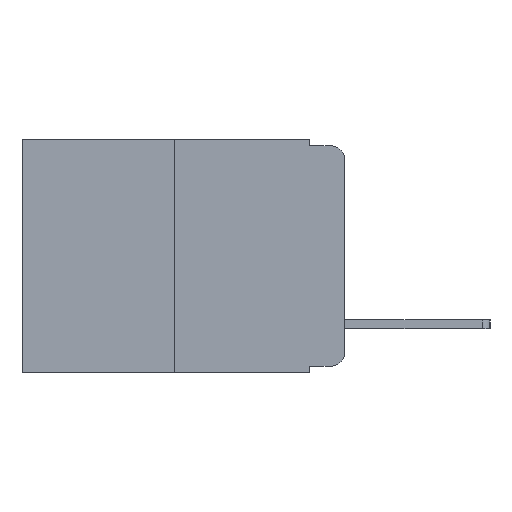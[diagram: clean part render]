
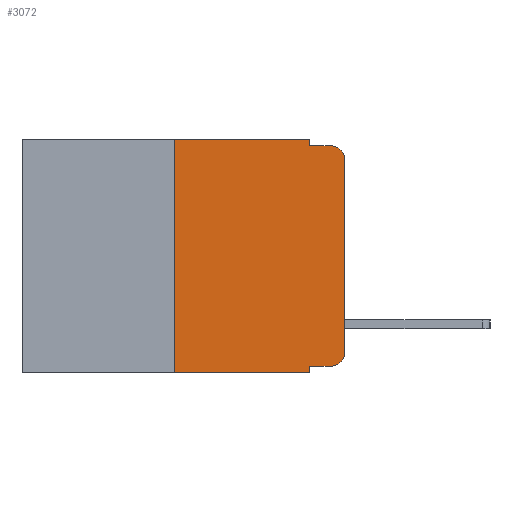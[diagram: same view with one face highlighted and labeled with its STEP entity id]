
A CAD part, left-side view. The second image highlights one B-rep face of the part: STEP entity #3072.
In plain terms, the highlighted planar face has unit normal (-1, 0, 0).
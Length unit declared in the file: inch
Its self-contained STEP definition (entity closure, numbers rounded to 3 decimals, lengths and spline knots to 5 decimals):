
#112 = CARTESIAN_POINT ( 'NONE',  ( 0., 0., -0.03 ) ) ;
#131 = DIRECTION ( 'NONE',  ( 0., 0., 1. ) ) ;
#229 = VECTOR ( 'NONE', #2544, 39.37008 ) ;
#315 = CARTESIAN_POINT ( 'NONE',  ( 0., 0.02, -0.03 ) ) ;
#396 = EDGE_CURVE ( 'NONE', #4921, #1701, #4086, .T. ) ;
#407 = CARTESIAN_POINT ( 'NONE',  ( 0., 0.25, -0.343 ) ) ;
#525 = ORIENTED_EDGE ( 'NONE', *, *, #9019, .T. ) ;
#843 = CARTESIAN_POINT ( 'NONE',  ( 0., 0.051, -0.333 ) ) ;
#1065 = CARTESIAN_POINT ( 'NONE',  ( 0., 0.051, 0. ) ) ;
#1195 = EDGE_CURVE ( 'NONE', #1701, #13211, #8880, .T. ) ;
#1236 = ORIENTED_EDGE ( 'NONE', *, *, #6186, .F. ) ;
#1292 = CARTESIAN_POINT ( 'NONE',  ( 0., 0.473, 0. ) ) ;
#1392 = CARTESIAN_POINT ( 'NONE',  ( 0., 0.02, -0.333 ) ) ;
#1486 = CARTESIAN_POINT ( 'NONE',  ( 0., 0.02, -0.313 ) ) ;
#1515 = DIRECTION ( 'NONE',  ( 0., 0., -1. ) ) ;
#1678 = AXIS2_PLACEMENT_3D ( 'NONE', #10008, #6788, #14211 ) ;
#1701 = VERTEX_POINT ( 'NONE', #2307 ) ;
#1955 = CARTESIAN_POINT ( 'NONE',  ( 0., 0.25, 0. ) ) ;
#2206 = ORIENTED_EDGE ( 'NONE', *, *, #3586, .T. ) ;
#2247 = EDGE_CURVE ( 'NONE', #2786, #3326, #3339, .T. ) ;
#2307 = CARTESIAN_POINT ( 'NONE',  ( 0., 0.051, -0.01 ) ) ;
#2544 = DIRECTION ( 'NONE',  ( 0., -1., 0. ) ) ;
#2578 = CARTESIAN_POINT ( 'NONE',  ( 0., 0.051, 0. ) ) ;
#2732 = DIRECTION ( 'NONE',  ( 0., 0., -1. ) ) ;
#2786 = VERTEX_POINT ( 'NONE', #407 ) ;
#2989 = ORIENTED_EDGE ( 'NONE', *, *, #10435, .T. ) ;
#3072 = ADVANCED_FACE ( 'NONE', ( #3471 ), #13159, .F. ) ;
#3326 = VERTEX_POINT ( 'NONE', #8492 ) ;
#3339 = LINE ( 'NONE', #4926, #13772 ) ;
#3471 = FACE_OUTER_BOUND ( 'NONE', #12791, .T. ) ;
#3476 = VERTEX_POINT ( 'NONE', #112 ) ;
#3586 = EDGE_CURVE ( 'NONE', #3476, #13211, #5196, .T. ) ;
#3739 = VECTOR ( 'NONE', #10333, 39.37008 ) ;
#3988 = ORIENTED_EDGE ( 'NONE', *, *, #396, .F. ) ;
#4086 = LINE ( 'NONE', #10873, #3739 ) ;
#4296 = VECTOR ( 'NONE', #131, 39.37008 ) ;
#4327 = EDGE_CURVE ( 'NONE', #4567, #3476, #13560, .T. ) ;
#4359 = DIRECTION ( 'NONE',  ( 0., -1., 0. ) ) ;
#4567 = VERTEX_POINT ( 'NONE', #8686 ) ;
#4624 = LINE ( 'NONE', #9177, #4296 ) ;
#4709 = VECTOR ( 'NONE', #4359, 39.37008 ) ;
#4794 = CARTESIAN_POINT ( 'NONE',  ( 0., 0.02, -0.01 ) ) ;
#4920 = AXIS2_PLACEMENT_3D ( 'NONE', #315, #8286, #1515 ) ;
#4921 = VERTEX_POINT ( 'NONE', #2578 ) ;
#4926 = CARTESIAN_POINT ( 'NONE',  ( 0., 0.473, -0.343 ) ) ;
#5191 = ORIENTED_EDGE ( 'NONE', *, *, #1195, .F. ) ;
#5196 = CIRCLE ( 'NONE', #4920, 0.02 ) ;
#6071 = CARTESIAN_POINT ( 'NONE',  ( 0., 0., 0. ) ) ;
#6186 = EDGE_CURVE ( 'NONE', #7967, #4921, #9248, .T. ) ;
#6581 = LINE ( 'NONE', #1065, #11925 ) ;
#6788 = DIRECTION ( 'NONE',  ( 1., 0., 0. ) ) ;
#6819 = VERTEX_POINT ( 'NONE', #8683 ) ;
#7164 = DIRECTION ( 'NONE',  ( 0., -1., 0. ) ) ;
#7628 = ORIENTED_EDGE ( 'NONE', *, *, #4327, .T. ) ;
#7665 = LINE ( 'NONE', #843, #4709 ) ;
#7967 = VERTEX_POINT ( 'NONE', #1955 ) ;
#8081 = DIRECTION ( 'NONE',  ( 0., -1., 0. ) ) ;
#8286 = DIRECTION ( 'NONE',  ( -1., 0., 0. ) ) ;
#8492 = CARTESIAN_POINT ( 'NONE',  ( 0., 0.051, -0.343 ) ) ;
#8683 = CARTESIAN_POINT ( 'NONE',  ( 0., 0.051, -0.333 ) ) ;
#8686 = CARTESIAN_POINT ( 'NONE',  ( 0., 0., -0.313 ) ) ;
#8880 = LINE ( 'NONE', #13311, #11673 ) ;
#9019 = EDGE_CURVE ( 'NONE', #11325, #4567, #9063, .T. ) ;
#9063 = CIRCLE ( 'NONE', #12712, 0.02 ) ;
#9177 = CARTESIAN_POINT ( 'NONE',  ( 0., 0.25, 0. ) ) ;
#9248 = LINE ( 'NONE', #1292, #229 ) ;
#9318 = DIRECTION ( 'NONE',  ( -1., 0., 0. ) ) ;
#9380 = DIRECTION ( 'NONE',  ( 0., 0., 1. ) ) ;
#10008 = CARTESIAN_POINT ( 'NONE',  ( 0., 0.473, 0. ) ) ;
#10133 = ORIENTED_EDGE ( 'NONE', *, *, #13227, .F. ) ;
#10333 = DIRECTION ( 'NONE',  ( 0., 0., -1. ) ) ;
#10435 = EDGE_CURVE ( 'NONE', #6819, #11325, #7665, .T. ) ;
#10873 = CARTESIAN_POINT ( 'NONE',  ( 0., 0.051, 0. ) ) ;
#11325 = VERTEX_POINT ( 'NONE', #1392 ) ;
#11673 = VECTOR ( 'NONE', #8081, 39.37008 ) ;
#11828 = EDGE_CURVE ( 'NONE', #6819, #3326, #6581, .T. ) ;
#11925 = VECTOR ( 'NONE', #13108, 39.37008 ) ;
#12712 = AXIS2_PLACEMENT_3D ( 'NONE', #1486, #9318, #2732 ) ;
#12791 = EDGE_LOOP ( 'NONE', ( #7628, #2206, #5191, #3988, #1236, #10133, #13254, #13771, #2989, #525 ) ) ;
#13108 = DIRECTION ( 'NONE',  ( 0., 0., -1. ) ) ;
#13159 = PLANE ( 'NONE',  #1678 ) ;
#13211 = VERTEX_POINT ( 'NONE', #4794 ) ;
#13221 = VECTOR ( 'NONE', #9380, 39.37008 ) ;
#13227 = EDGE_CURVE ( 'NONE', #2786, #7967, #4624, .T. ) ;
#13254 = ORIENTED_EDGE ( 'NONE', *, *, #2247, .T. ) ;
#13311 = CARTESIAN_POINT ( 'NONE',  ( 0., 0.051, -0.01 ) ) ;
#13560 = LINE ( 'NONE', #6071, #13221 ) ;
#13771 = ORIENTED_EDGE ( 'NONE', *, *, #11828, .F. ) ;
#13772 = VECTOR ( 'NONE', #7164, 39.37008 ) ;
#14211 = DIRECTION ( 'NONE',  ( 0., 0., -1. ) ) ;
